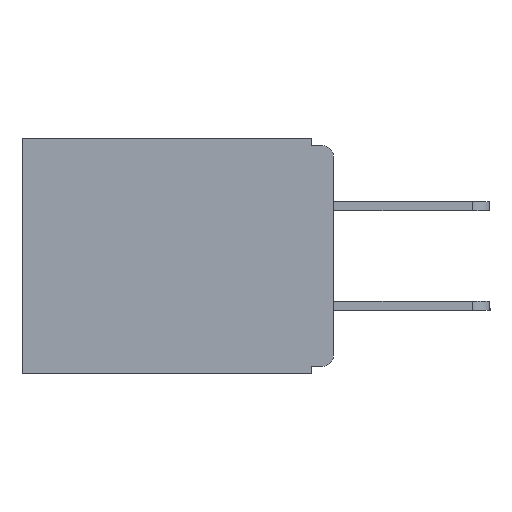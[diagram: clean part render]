
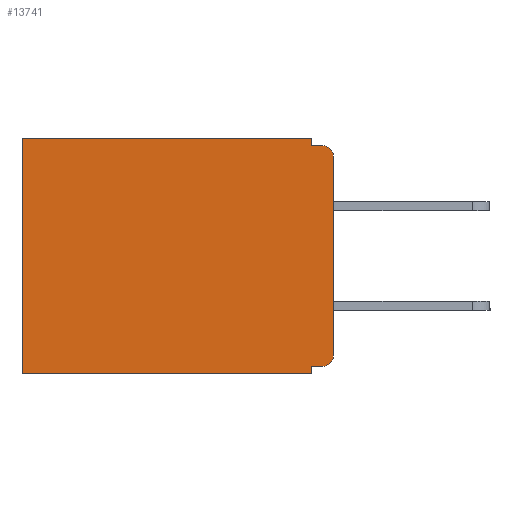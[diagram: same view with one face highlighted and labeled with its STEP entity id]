
A CAD part, left-side view. The second image highlights one B-rep face of the part: STEP entity #13741.
In plain terms, the highlighted planar face has unit normal (-1, 0, 0).
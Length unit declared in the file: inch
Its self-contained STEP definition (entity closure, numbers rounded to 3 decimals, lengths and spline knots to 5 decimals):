
#38 = LINE ( 'NONE', #17332, #11122 ) ;
#248 = LINE ( 'NONE', #13065, #18105 ) ;
#325 = CARTESIAN_POINT ( 'NONE',  ( 0.3, 0.015, -0.32 ) ) ;
#404 = CIRCLE ( 'NONE', #10559, 0.015 ) ;
#815 = ORIENTED_EDGE ( 'NONE', *, *, #5962, .F. ) ;
#920 = DIRECTION ( 'NONE',  ( 1., 0., 0. ) ) ;
#1311 = LINE ( 'NONE', #8109, #5215 ) ;
#1428 = VERTEX_POINT ( 'NONE', #1513 ) ;
#1510 = CARTESIAN_POINT ( 'NONE',  ( 0.3, 0.437, 0. ) ) ;
#1513 = CARTESIAN_POINT ( 'NONE',  ( 0.3, 0.031, -0.32 ) ) ;
#1979 = LINE ( 'NONE', #9387, #5441 ) ;
#2090 = ORIENTED_EDGE ( 'NONE', *, *, #9786, .T. ) ;
#2139 = ORIENTED_EDGE ( 'NONE', *, *, #3511, .F. ) ;
#2176 = DIRECTION ( 'NONE',  ( 0., 1., 0. ) ) ;
#2239 = CARTESIAN_POINT ( 'NONE',  ( 0.3, 0., 0. ) ) ;
#2271 = DIRECTION ( 'NONE',  ( 0., 0., -1. ) ) ;
#2314 = DIRECTION ( 'NONE',  ( -1., 0., 0. ) ) ;
#2343 = CARTESIAN_POINT ( 'NONE',  ( 0.3, 0.015, -0.305 ) ) ;
#2962 = VECTOR ( 'NONE', #13378, 39.37008 ) ;
#3037 = CARTESIAN_POINT ( 'NONE',  ( 0.3, 0.031, -0.33 ) ) ;
#3511 = EDGE_CURVE ( 'NONE', #5337, #1428, #38, .T. ) ;
#4027 = EDGE_CURVE ( 'NONE', #5184, #8478, #248, .T. ) ;
#4076 = DIRECTION ( 'NONE',  ( 0., 1., 0. ) ) ;
#4337 = VERTEX_POINT ( 'NONE', #15067 ) ;
#4440 = CARTESIAN_POINT ( 'NONE',  ( 0.3, 0.015, -0.025 ) ) ;
#4454 = LINE ( 'NONE', #2239, #7860 ) ;
#5089 = ORIENTED_EDGE ( 'NONE', *, *, #6123, .F. ) ;
#5184 = VERTEX_POINT ( 'NONE', #1510 ) ;
#5215 = VECTOR ( 'NONE', #8280, 39.37008 ) ;
#5337 = VERTEX_POINT ( 'NONE', #325 ) ;
#5423 = ORIENTED_EDGE ( 'NONE', *, *, #6837, .T. ) ;
#5441 = VECTOR ( 'NONE', #12168, 39.37008 ) ;
#5449 = DIRECTION ( 'NONE',  ( 0., 0., -1. ) ) ;
#5909 = DIRECTION ( 'NONE',  ( 0., 0., -1. ) ) ;
#5962 = EDGE_CURVE ( 'NONE', #11707, #8478, #11060, .T. ) ;
#5976 = ORIENTED_EDGE ( 'NONE', *, *, #4027, .T. ) ;
#6123 = EDGE_CURVE ( 'NONE', #4337, #10723, #15328, .T. ) ;
#6494 = ORIENTED_EDGE ( 'NONE', *, *, #12997, .F. ) ;
#6824 = CARTESIAN_POINT ( 'NONE',  ( 0.3, 0., -0.33 ) ) ;
#6837 = EDGE_CURVE ( 'NONE', #5337, #8480, #404, .T. ) ;
#6935 = ORIENTED_EDGE ( 'NONE', *, *, #7709, .F. ) ;
#7551 = VECTOR ( 'NONE', #7602, 39.37008 ) ;
#7602 = DIRECTION ( 'NONE',  ( 0., -1., 0. ) ) ;
#7709 = EDGE_CURVE ( 'NONE', #14757, #8480, #1311, .T. ) ;
#7860 = VECTOR ( 'NONE', #2176, 39.37008 ) ;
#8109 = CARTESIAN_POINT ( 'NONE',  ( 0.3, 0., -0.33 ) ) ;
#8210 = CARTESIAN_POINT ( 'NONE',  ( 0.3, 0., -0.33 ) ) ;
#8280 = DIRECTION ( 'NONE',  ( 0., 0., -1. ) ) ;
#8478 = VERTEX_POINT ( 'NONE', #14647 ) ;
#8480 = VERTEX_POINT ( 'NONE', #14338 ) ;
#8551 = CARTESIAN_POINT ( 'NONE',  ( 0.3, 0.031, 0. ) ) ;
#9268 = AXIS2_PLACEMENT_3D ( 'NONE', #4440, #14254, #5909 ) ;
#9363 = EDGE_LOOP ( 'NONE', ( #6935, #14971, #5089, #6494, #2090, #5976, #815, #12705, #2139, #5423 ) ) ;
#9387 = CARTESIAN_POINT ( 'NONE',  ( 0.3, 0.031, 0. ) ) ;
#9786 = EDGE_CURVE ( 'NONE', #17654, #5184, #4454, .T. ) ;
#10227 = DIRECTION ( 'NONE',  ( 0., 0., -1. ) ) ;
#10559 = AXIS2_PLACEMENT_3D ( 'NONE', #2343, #2314, #2271 ) ;
#10723 = VERTEX_POINT ( 'NONE', #11569 ) ;
#11003 = DIRECTION ( 'NONE',  ( 0., 0., -1. ) ) ;
#11060 = LINE ( 'NONE', #6824, #2962 ) ;
#11122 = VECTOR ( 'NONE', #4076, 39.37008 ) ;
#11268 = CARTESIAN_POINT ( 'NONE',  ( 0.3, 0., -0.01 ) ) ;
#11569 = CARTESIAN_POINT ( 'NONE',  ( 0.3, 0.015, -0.01 ) ) ;
#11707 = VERTEX_POINT ( 'NONE', #14052 ) ;
#12168 = DIRECTION ( 'NONE',  ( 0., 0., -1. ) ) ;
#12414 = LINE ( 'NONE', #3037, #16429 ) ;
#12475 = EDGE_CURVE ( 'NONE', #14757, #10723, #18219, .T. ) ;
#12705 = ORIENTED_EDGE ( 'NONE', *, *, #15151, .F. ) ;
#12997 = EDGE_CURVE ( 'NONE', #17654, #4337, #1979, .T. ) ;
#13065 = CARTESIAN_POINT ( 'NONE',  ( 0.3, 0.437, -0.33 ) ) ;
#13378 = DIRECTION ( 'NONE',  ( 0., 1., 0. ) ) ;
#13741 = ADVANCED_FACE ( 'NONE', ( #18173 ), #16410, .F. ) ;
#14052 = CARTESIAN_POINT ( 'NONE',  ( 0.3, 0.031, -0.33 ) ) ;
#14254 = DIRECTION ( 'NONE',  ( -1., 0., 0. ) ) ;
#14338 = CARTESIAN_POINT ( 'NONE',  ( 0.3, 0., -0.305 ) ) ;
#14647 = CARTESIAN_POINT ( 'NONE',  ( 0.3, 0.437, -0.33 ) ) ;
#14757 = VERTEX_POINT ( 'NONE', #17558 ) ;
#14971 = ORIENTED_EDGE ( 'NONE', *, *, #12475, .T. ) ;
#15067 = CARTESIAN_POINT ( 'NONE',  ( 0.3, 0.031, -0.01 ) ) ;
#15151 = EDGE_CURVE ( 'NONE', #1428, #11707, #12414, .T. ) ;
#15328 = LINE ( 'NONE', #11268, #7551 ) ;
#16410 = PLANE ( 'NONE',  #17967 ) ;
#16429 = VECTOR ( 'NONE', #10227, 39.37008 ) ;
#17332 = CARTESIAN_POINT ( 'NONE',  ( 0.3, 0., -0.32 ) ) ;
#17558 = CARTESIAN_POINT ( 'NONE',  ( 0.3, 0., -0.025 ) ) ;
#17654 = VERTEX_POINT ( 'NONE', #8551 ) ;
#17967 = AXIS2_PLACEMENT_3D ( 'NONE', #8210, #920, #11003 ) ;
#18105 = VECTOR ( 'NONE', #5449, 39.37008 ) ;
#18173 = FACE_OUTER_BOUND ( 'NONE', #9363, .T. ) ;
#18219 = CIRCLE ( 'NONE', #9268, 0.015 ) ;
